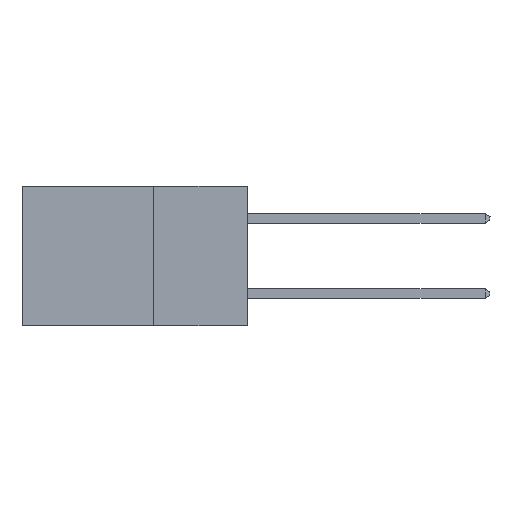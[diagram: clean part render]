
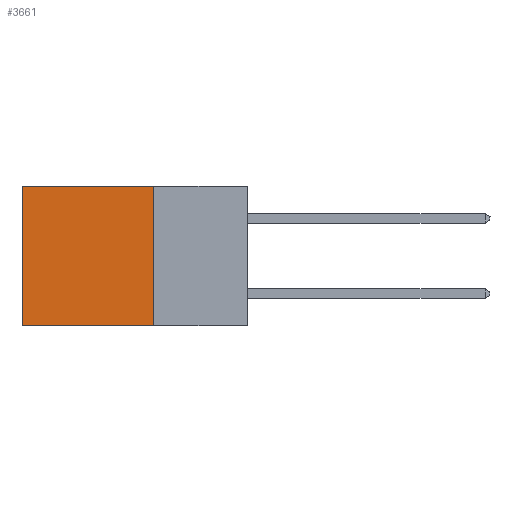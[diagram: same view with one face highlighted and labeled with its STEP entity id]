
A CAD part, left-side view. The second image highlights one B-rep face of the part: STEP entity #3661.
In plain terms, the highlighted planar face has unit normal (-1, 0, 0).
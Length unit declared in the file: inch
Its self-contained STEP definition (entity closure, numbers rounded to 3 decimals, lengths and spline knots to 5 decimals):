
#50 = VERTEX_POINT ( 'NONE', #3933 ) ;
#2278 = EDGE_CURVE ( 'NONE', #50, #22257, #25702, .T. ) ;
#2787 = PLANE ( 'NONE',  #19192 ) ;
#3661 = ADVANCED_FACE ( 'NONE', ( #25703 ), #2787, .F. ) ;
#3933 = CARTESIAN_POINT ( 'NONE',  ( 0.298, 0.25, -0.37 ) ) ;
#4552 = EDGE_CURVE ( 'NONE', #15228, #22257, #19796, .T. ) ;
#4811 = DIRECTION ( 'NONE',  ( 0., 1., 0. ) ) ;
#5615 = CARTESIAN_POINT ( 'NONE',  ( 0.298, 0.25, 0. ) ) ;
#5681 = DIRECTION ( 'NONE',  ( 0., 0., -1. ) ) ;
#6812 = EDGE_CURVE ( 'NONE', #29201, #15228, #25119, .T. ) ;
#7211 = VECTOR ( 'NONE', #5681, 39.37008 ) ;
#7784 = CARTESIAN_POINT ( 'NONE',  ( 0.298, 0.25, 0. ) ) ;
#7991 = ORIENTED_EDGE ( 'NONE', *, *, #13720, .F. ) ;
#8331 = DIRECTION ( 'NONE',  ( 1., 0., 0. ) ) ;
#10674 = CARTESIAN_POINT ( 'NONE',  ( 0.298, 0.6, -0.37 ) ) ;
#12640 = VECTOR ( 'NONE', #28286, 39.37008 ) ;
#13720 = EDGE_CURVE ( 'NONE', #29201, #50, #17459, .T. ) ;
#14828 = CARTESIAN_POINT ( 'NONE',  ( 0.298, 0.6, 0. ) ) ;
#15228 = VERTEX_POINT ( 'NONE', #15477 ) ;
#15477 = CARTESIAN_POINT ( 'NONE',  ( 0.298, 0.6, 0. ) ) ;
#16717 = VECTOR ( 'NONE', #22131, 39.37008 ) ;
#17064 = ORIENTED_EDGE ( 'NONE', *, *, #4552, .T. ) ;
#17459 = LINE ( 'NONE', #5615, #16717 ) ;
#17690 = EDGE_LOOP ( 'NONE', ( #17064, #18197, #7991, #21678 ) ) ;
#18197 = ORIENTED_EDGE ( 'NONE', *, *, #2278, .F. ) ;
#18506 = CARTESIAN_POINT ( 'NONE',  ( 0.298, 0.25, 0. ) ) ;
#19192 = AXIS2_PLACEMENT_3D ( 'NONE', #18506, #8331, #28528 ) ;
#19489 = VECTOR ( 'NONE', #4811, 39.37008 ) ;
#19796 = LINE ( 'NONE', #14828, #7211 ) ;
#21678 = ORIENTED_EDGE ( 'NONE', *, *, #6812, .T. ) ;
#22131 = DIRECTION ( 'NONE',  ( 0., 0., -1. ) ) ;
#22257 = VERTEX_POINT ( 'NONE', #10674 ) ;
#23013 = CARTESIAN_POINT ( 'NONE',  ( 0.298, 0.25, -0.37 ) ) ;
#25119 = LINE ( 'NONE', #28369, #12640 ) ;
#25702 = LINE ( 'NONE', #23013, #19489 ) ;
#25703 = FACE_OUTER_BOUND ( 'NONE', #17690, .T. ) ;
#28286 = DIRECTION ( 'NONE',  ( 0., 1., 0. ) ) ;
#28369 = CARTESIAN_POINT ( 'NONE',  ( 0.298, 0.25, 0. ) ) ;
#28528 = DIRECTION ( 'NONE',  ( 0., 0., -1. ) ) ;
#29201 = VERTEX_POINT ( 'NONE', #7784 ) ;
